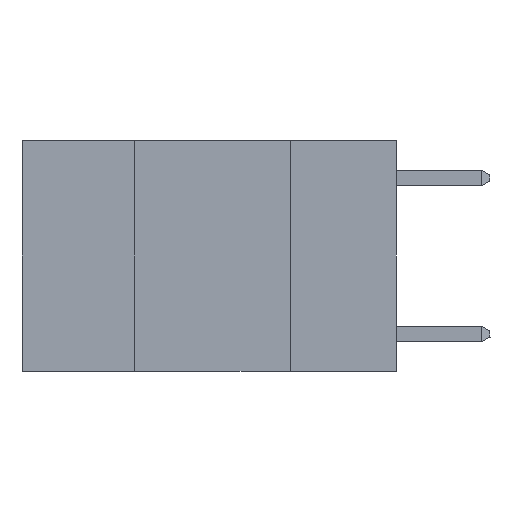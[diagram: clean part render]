
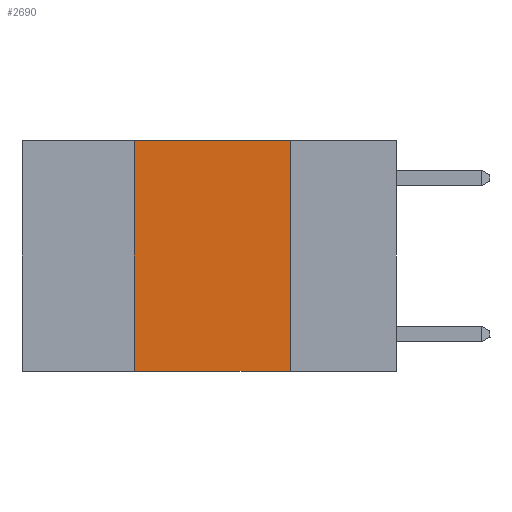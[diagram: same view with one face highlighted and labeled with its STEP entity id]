
A CAD part, left-side view. The second image highlights one B-rep face of the part: STEP entity #2690.
In plain terms, the highlighted planar face has unit normal (-1, 0, 0).
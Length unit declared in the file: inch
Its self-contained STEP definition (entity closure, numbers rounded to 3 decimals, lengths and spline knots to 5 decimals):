
#218 = DIRECTION ( 'NONE',  ( 1., 0., 0. ) ) ;
#1455 = DIRECTION ( 'NONE',  ( 0., 0., -1. ) ) ;
#1790 = EDGE_CURVE ( 'NONE', #16705, #12692, #9089, .T. ) ;
#2357 = DIRECTION ( 'NONE',  ( 0., -1., 0. ) ) ;
#2690 = ADVANCED_FACE ( 'NONE', ( #25078 ), #11898, .F. ) ;
#2878 = CARTESIAN_POINT ( 'NONE',  ( 0., 0.42, -0.37 ) ) ;
#5057 = CARTESIAN_POINT ( 'NONE',  ( 0., 0.42, 0. ) ) ;
#6040 = CARTESIAN_POINT ( 'NONE',  ( 0., 0.6, 0. ) ) ;
#6332 = ORIENTED_EDGE ( 'NONE', *, *, #19243, .T. ) ;
#7296 = VERTEX_POINT ( 'NONE', #2878 ) ;
#8462 = VECTOR ( 'NONE', #2357, 39.37008 ) ;
#9089 = LINE ( 'NONE', #13121, #14254 ) ;
#10281 = ORIENTED_EDGE ( 'NONE', *, *, #1790, .F. ) ;
#11364 = DIRECTION ( 'NONE',  ( 0., 0., 1. ) ) ;
#11736 = DIRECTION ( 'NONE',  ( 0., -1., 0. ) ) ;
#11880 = VECTOR ( 'NONE', #11364, 39.37008 ) ;
#11898 = PLANE ( 'NONE',  #24934 ) ;
#11998 = VECTOR ( 'NONE', #11736, 39.37008 ) ;
#12692 = VERTEX_POINT ( 'NONE', #16459 ) ;
#13121 = CARTESIAN_POINT ( 'NONE',  ( 0., 0.17, 0. ) ) ;
#13470 = CARTESIAN_POINT ( 'NONE',  ( 0., 0.6, -0.37 ) ) ;
#13627 = LINE ( 'NONE', #23664, #8462 ) ;
#13866 = DIRECTION ( 'NONE',  ( 0., 0., -1. ) ) ;
#14254 = VECTOR ( 'NONE', #1455, 39.37008 ) ;
#15529 = CARTESIAN_POINT ( 'NONE',  ( 0., 0.17, 0. ) ) ;
#16073 = ORIENTED_EDGE ( 'NONE', *, *, #23098, .F. ) ;
#16459 = CARTESIAN_POINT ( 'NONE',  ( 0., 0.17, -0.37 ) ) ;
#16705 = VERTEX_POINT ( 'NONE', #15529 ) ;
#17191 = LINE ( 'NONE', #13470, #11998 ) ;
#17244 = CARTESIAN_POINT ( 'NONE',  ( 0., 0.42, 0. ) ) ;
#18242 = VERTEX_POINT ( 'NONE', #5057 ) ;
#19243 = EDGE_CURVE ( 'NONE', #7296, #12692, #17191, .T. ) ;
#20599 = ORIENTED_EDGE ( 'NONE', *, *, #24900, .F. ) ;
#21553 = EDGE_LOOP ( 'NONE', ( #10281, #20599, #16073, #6332 ) ) ;
#22176 = LINE ( 'NONE', #17244, #11880 ) ;
#23098 = EDGE_CURVE ( 'NONE', #7296, #18242, #22176, .T. ) ;
#23664 = CARTESIAN_POINT ( 'NONE',  ( 0., 0.6, 0. ) ) ;
#24900 = EDGE_CURVE ( 'NONE', #18242, #16705, #13627, .T. ) ;
#24934 = AXIS2_PLACEMENT_3D ( 'NONE', #6040, #218, #13866 ) ;
#25078 = FACE_OUTER_BOUND ( 'NONE', #21553, .T. ) ;
